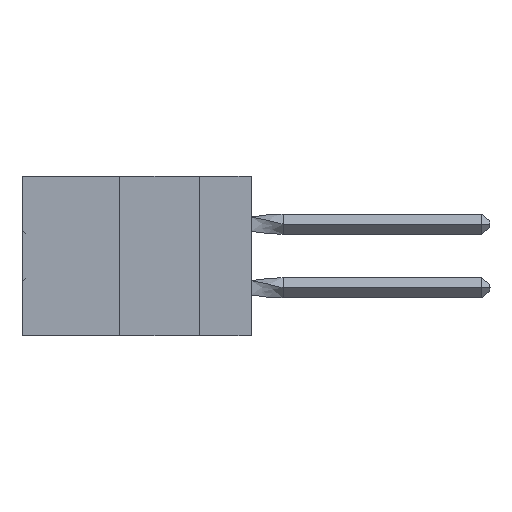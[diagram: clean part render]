
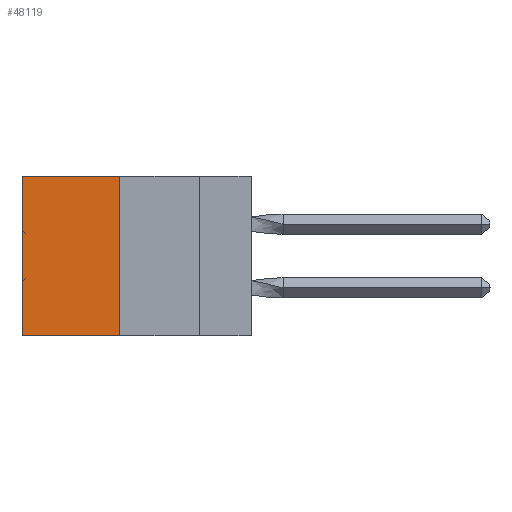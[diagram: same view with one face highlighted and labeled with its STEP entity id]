
A CAD part, left-side view. The second image highlights one B-rep face of the part: STEP entity #48119.
In plain terms, the highlighted planar face has unit normal (-1, 0, 0).
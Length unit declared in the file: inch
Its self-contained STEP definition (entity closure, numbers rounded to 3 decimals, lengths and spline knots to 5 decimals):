
#572 = DIRECTION ( 'NONE',  ( 0., 0., -1. ) ) ;
#3503 = CARTESIAN_POINT ( 'NONE',  ( 0.305, 0.72, -0.5 ) ) ;
#4336 = EDGE_LOOP ( 'NONE', ( #57675, #26745, #14131, #8422 ) ) ;
#6188 = VECTOR ( 'NONE', #22854, 39.37008 ) ;
#7741 = AXIS2_PLACEMENT_3D ( 'NONE', #53205, #39354, #52399 ) ;
#8396 = CARTESIAN_POINT ( 'NONE',  ( 0.305, 0.413, -0.5 ) ) ;
#8422 = ORIENTED_EDGE ( 'NONE', *, *, #27442, .T. ) ;
#14131 = ORIENTED_EDGE ( 'NONE', *, *, #19568, .F. ) ;
#15329 = EDGE_CURVE ( 'NONE', #24814, #18808, #56006, .T. ) ;
#18785 = LINE ( 'NONE', #8396, #58163 ) ;
#18808 = VERTEX_POINT ( 'NONE', #3503 ) ;
#19568 = EDGE_CURVE ( 'NONE', #28594, #24814, #18785, .T. ) ;
#22687 = EDGE_CURVE ( 'NONE', #54896, #18808, #27552, .T. ) ;
#22776 = CARTESIAN_POINT ( 'NONE',  ( 0.305, 0.72, -0.5 ) ) ;
#22854 = DIRECTION ( 'NONE',  ( 0., 1., 0. ) ) ;
#24705 = CARTESIAN_POINT ( 'NONE',  ( 0.305, 0.413, -0.5 ) ) ;
#24814 = VERTEX_POINT ( 'NONE', #36298 ) ;
#26745 = ORIENTED_EDGE ( 'NONE', *, *, #15329, .F. ) ;
#27442 = EDGE_CURVE ( 'NONE', #28594, #54896, #45570, .T. ) ;
#27552 = LINE ( 'NONE', #22776, #34014 ) ;
#28594 = VERTEX_POINT ( 'NONE', #30597 ) ;
#30597 = CARTESIAN_POINT ( 'NONE',  ( 0.305, 0.413, 0. ) ) ;
#31620 = DIRECTION ( 'NONE',  ( 0., 0., -1. ) ) ;
#34014 = VECTOR ( 'NONE', #572, 39.37008 ) ;
#36298 = CARTESIAN_POINT ( 'NONE',  ( 0.305, 0.413, -0.5 ) ) ;
#39354 = DIRECTION ( 'NONE',  ( 1., 0., 0. ) ) ;
#43693 = FACE_OUTER_BOUND ( 'NONE', #4336, .T. ) ;
#43851 = VECTOR ( 'NONE', #57293, 39.37008 ) ;
#45570 = LINE ( 'NONE', #59069, #6188 ) ;
#48119 = ADVANCED_FACE ( 'NONE', ( #43693 ), #52602, .F. ) ;
#52399 = DIRECTION ( 'NONE',  ( 0., 0., -1. ) ) ;
#52602 = PLANE ( 'NONE',  #7741 ) ;
#53205 = CARTESIAN_POINT ( 'NONE',  ( 0.305, 0.413, -0.5 ) ) ;
#54896 = VERTEX_POINT ( 'NONE', #56835 ) ;
#56006 = LINE ( 'NONE', #24705, #43851 ) ;
#56835 = CARTESIAN_POINT ( 'NONE',  ( 0.305, 0.72, 0. ) ) ;
#57293 = DIRECTION ( 'NONE',  ( 0., 1., 0. ) ) ;
#57675 = ORIENTED_EDGE ( 'NONE', *, *, #22687, .T. ) ;
#58163 = VECTOR ( 'NONE', #31620, 39.37008 ) ;
#59069 = CARTESIAN_POINT ( 'NONE',  ( 0.305, 0.413, 0. ) ) ;
